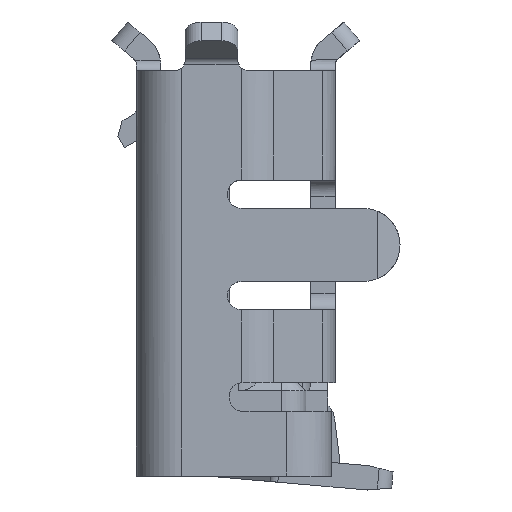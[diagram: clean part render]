
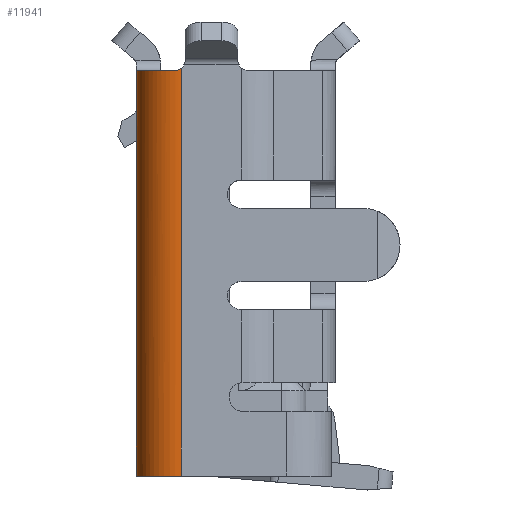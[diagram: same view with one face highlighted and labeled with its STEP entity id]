
A CAD part, left-side view. The second image highlights one B-rep face of the part: STEP entity #11941.
In plain terms, the highlighted cylindrical face has radius 0.55 mm (diameter 1.1 mm), a partial arc.
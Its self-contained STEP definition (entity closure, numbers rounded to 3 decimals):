
#189 = CARTESIAN_POINT ( 'NONE',  ( 3.715, -3.5, -0.878 ) ) ;
#538 = CARTESIAN_POINT ( 'NONE',  ( 3.75, 1.5, -0.675 ) ) ;
#749 = CARTESIAN_POINT ( 'NONE',  ( 3.75, 1.5, -0.675 ) ) ;
#836 = CARTESIAN_POINT ( 'NONE',  ( 3.2, -3.502, -1.225 ) ) ;
#1075 = CARTESIAN_POINT ( 'NONE',  ( 3.2, 1.5, -1.225 ) ) ;
#1309 = B_SPLINE_CURVE_WITH_KNOTS ( 'NONE', 3,
 ( #836, #11412, #2698, #8005 ),
 .UNSPECIFIED., .F., .F.,
 ( 4, 4 ),
 ( 0., 1. ),
 .UNSPECIFIED. ) ;
#1439 = ORIENTED_EDGE ( 'NONE', *, *, #5905, .F. ) ;
#1597 = CARTESIAN_POINT ( 'NONE',  ( 3.735, -3.5, -0.818 ) ) ;
#2038 = CARTESIAN_POINT ( 'NONE',  ( 3.733, 1.5, -0.817 ) ) ;
#2503 = CARTESIAN_POINT ( 'NONE',  ( 3.477, 1.5, -1.152 ) ) ;
#2527 = CARTESIAN_POINT ( 'NONE',  ( 3.2, 1.5, -0.675 ) ) ;
#2698 = CARTESIAN_POINT ( 'NONE',  ( 3.22, -3.5, -1.225 ) ) ;
#2805 = ORIENTED_EDGE ( 'NONE', *, *, #11868, .F. ) ;
#3812 = CARTESIAN_POINT ( 'NONE',  ( 3.444, 1.5, -1.169 ) ) ;
#4048 = CARTESIAN_POINT ( 'NONE',  ( 3.678, 1.5, -0.95 ) ) ;
#4273 = FACE_OUTER_BOUND ( 'NONE', #20687, .T. ) ;
#4499 = ORIENTED_EDGE ( 'NONE', *, *, #13460, .F. ) ;
#5250 = VECTOR ( 'NONE', #15812, 1000. ) ;
#5565 = CARTESIAN_POINT ( 'NONE',  ( 3.344, 1.5, -1.211 ) ) ;
#5597 = CARTESIAN_POINT ( 'NONE',  ( 3.2, -1.035, -1.225 ) ) ;
#5685 = CARTESIAN_POINT ( 'NONE',  ( 3.564, 1.5, -1.089 ) ) ;
#5905 = EDGE_CURVE ( 'NONE', #12017, #20618, #7471, .T. ) ;
#6041 = CARTESIAN_POINT ( 'NONE',  ( 3.2, 1.5, -1.225 ) ) ;
#6272 = VERTEX_POINT ( 'NONE', #749 ) ;
#7096 = CARTESIAN_POINT ( 'NONE',  ( 3.744, -3.5, -0.755 ) ) ;
#7116 = CARTESIAN_POINT ( 'NONE',  ( 3.617, -3.5, -1.04 ) ) ;
#7233 = CARTESIAN_POINT ( 'NONE',  ( 3.656, -3.5, -0.988 ) ) ;
#7396 = CARTESIAN_POINT ( 'NONE',  ( 3.75, -3.528, -0.675 ) ) ;
#7471 = B_SPLINE_CURVE_WITH_KNOTS ( 'NONE', 3,
 ( #23176, #14264, #18009, #10243, #23049, #12523, #17889, #7116, #7233, #189, #1597, #14494 ),
 .UNSPECIFIED., .F., .F.,
 ( 4, 2, 2, 2, 2, 4 ),
 ( 0., 0.25, 0.375, 0.5, 0.75, 1. ),
 .UNSPECIFIED. ) ;
#7583 = CARTESIAN_POINT ( 'NONE',  ( 3.695, 1.5, -0.918 ) ) ;
#7691 = CARTESIAN_POINT ( 'NONE',  ( 3.614, 1.5, -1.039 ) ) ;
#8005 = CARTESIAN_POINT ( 'NONE',  ( 3.23, -3.5, -1.224 ) ) ;
#8677 = LINE ( 'NONE', #5597, #5250 ) ;
#8924 = B_SPLINE_CURVE_WITH_KNOTS ( 'NONE', 3,
 ( #538, #19887, #14952, #2038, #13207, #7583, #4048, #19997, #7691, #5685, #16340, #2503, #3812, #5565, #12859, #6041 ),
 .UNSPECIFIED., .F., .F.,
 ( 4, 2, 2, 2, 2, 2, 2, 4 ),
 ( 0., 0.125, 0.25, 0.375, 0.5, 0.625, 0.75, 1. ),
 .UNSPECIFIED. ) ;
#9540 = ORIENTED_EDGE ( 'NONE', *, *, #19093, .T. ) ;
#9833 = LINE ( 'NONE', #18365, #12682 ) ;
#10243 = CARTESIAN_POINT ( 'NONE',  ( 3.441, -3.5, -1.17 ) ) ;
#10591 = ORIENTED_EDGE ( 'NONE', *, *, #21714, .F. ) ;
#11189 = CARTESIAN_POINT ( 'NONE',  ( 3.744, -3.5, -0.755 ) ) ;
#11363 = DIRECTION ( 'NONE',  ( 0., 1., 0. ) ) ;
#11412 = CARTESIAN_POINT ( 'NONE',  ( 3.21, -3.501, -1.225 ) ) ;
#11868 = EDGE_CURVE ( 'NONE', #18727, #6272, #9833, .T. ) ;
#11886 = CARTESIAN_POINT ( 'NONE',  ( 3.2, -3.502, -1.225 ) ) ;
#11911 = B_SPLINE_CURVE_WITH_KNOTS ( 'NONE', 3,
 ( #7096, #21499, #22056, #13175 ),
 .UNSPECIFIED., .F., .F.,
 ( 4, 4 ),
 ( 0., 1. ),
 .UNSPECIFIED. ) ;
#11941 = ADVANCED_FACE ( 'NONE', ( #4273 ), #18718, .T. ) ;
#12017 = VERTEX_POINT ( 'NONE', #19408 ) ;
#12523 = CARTESIAN_POINT ( 'NONE',  ( 3.522, -3.5, -1.122 ) ) ;
#12682 = VECTOR ( 'NONE', #11363, 1000. ) ;
#12859 = CARTESIAN_POINT ( 'NONE',  ( 3.274, 1.5, -1.225 ) ) ;
#13175 = CARTESIAN_POINT ( 'NONE',  ( 3.75, -3.528, -0.675 ) ) ;
#13207 = CARTESIAN_POINT ( 'NONE',  ( 3.722, 1.5, -0.852 ) ) ;
#13332 = DIRECTION ( 'NONE',  ( 0., 0., -1. ) ) ;
#13460 = EDGE_CURVE ( 'NONE', #15550, #12017, #1309, .T. ) ;
#14264 = CARTESIAN_POINT ( 'NONE',  ( 3.293, -3.5, -1.221 ) ) ;
#14494 = CARTESIAN_POINT ( 'NONE',  ( 3.744, -3.5, -0.755 ) ) ;
#14952 = CARTESIAN_POINT ( 'NONE',  ( 3.747, 1.5, -0.747 ) ) ;
#15550 = VERTEX_POINT ( 'NONE', #11886 ) ;
#15812 = DIRECTION ( 'NONE',  ( 0., 1., 0. ) ) ;
#16340 = CARTESIAN_POINT ( 'NONE',  ( 3.536, 1.5, -1.112 ) ) ;
#16602 = DIRECTION ( 'NONE',  ( 0., -1., 0. ) ) ;
#17889 = CARTESIAN_POINT ( 'NONE',  ( 3.548, -3.5, -1.102 ) ) ;
#18009 = CARTESIAN_POINT ( 'NONE',  ( 3.355, -3.5, -1.206 ) ) ;
#18265 = AXIS2_PLACEMENT_3D ( 'NONE', #2527, #16602, #13332 ) ;
#18365 = CARTESIAN_POINT ( 'NONE',  ( 3.75, -1.014, -0.675 ) ) ;
#18569 = ORIENTED_EDGE ( 'NONE', *, *, #19621, .F. ) ;
#18718 = CYLINDRICAL_SURFACE ( 'NONE', #18265, 0.55 ) ;
#18727 = VERTEX_POINT ( 'NONE', #7396 ) ;
#19093 = EDGE_CURVE ( 'NONE', #15550, #20666, #8677, .T. ) ;
#19408 = CARTESIAN_POINT ( 'NONE',  ( 3.23, -3.5, -1.224 ) ) ;
#19621 = EDGE_CURVE ( 'NONE', #6272, #20666, #8924, .T. ) ;
#19887 = CARTESIAN_POINT ( 'NONE',  ( 3.75, 1.5, -0.711 ) ) ;
#19997 = CARTESIAN_POINT ( 'NONE',  ( 3.638, 1.5, -1.009 ) ) ;
#20618 = VERTEX_POINT ( 'NONE', #11189 ) ;
#20666 = VERTEX_POINT ( 'NONE', #1075 ) ;
#20687 = EDGE_LOOP ( 'NONE', ( #4499, #9540, #18569, #2805, #10591, #1439 ) ) ;
#21499 = CARTESIAN_POINT ( 'NONE',  ( 3.748, -3.5, -0.728 ) ) ;
#21714 = EDGE_CURVE ( 'NONE', #20618, #18727, #11911, .T. ) ;
#22056 = CARTESIAN_POINT ( 'NONE',  ( 3.75, -3.508, -0.699 ) ) ;
#23049 = CARTESIAN_POINT ( 'NONE',  ( 3.469, -3.5, -1.156 ) ) ;
#23176 = CARTESIAN_POINT ( 'NONE',  ( 3.23, -3.5, -1.224 ) ) ;
